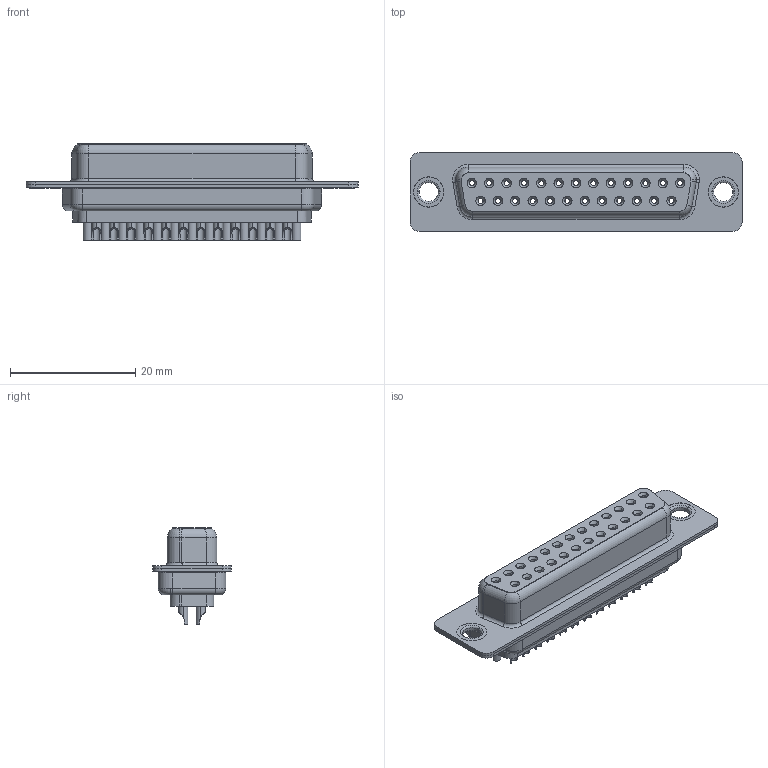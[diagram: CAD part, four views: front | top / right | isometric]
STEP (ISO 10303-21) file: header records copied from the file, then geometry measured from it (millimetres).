
FILE_DESCRIPTION (( 'STEP AP203' ), '1' );
FILE_NAME ('628-025-622-061.STEP', '2020-07-14T15:30:57', ( '' ), ( '' ), 'SwSTEP 2.0', 'SolidWorks 2020', '' );
FILE_SCHEMA (( 'CONFIG_CONTROL_DESIGN' ));
Length unit declared in the file: millimetre
Products named in the file (7): 628 Thru Hole Rivet; 628 Contact Row 2_22L; 628 Housing_25 LP; 628-025-622-061; 628 Contact Row 1_22L; 628 Shell Front_25 Contacts; 628 Shell Rear_25 Contacts
Assembly tree (30 placements, depth 2):
  628-025-622-061
    628 Housing_25 LP
    628 Shell Front_25 Contacts
    628 Shell Rear_25 Contacts
    628 Contact Row 1_22L  x13
    628 Contact Row 2_22L  x12
    628 Thru Hole Rivet  x2
Bounding box: 53 x 12.6 x 15.35 mm (x, y, z)
Volume: 3766.9 mm3; surface area: 9245.1 mm2
Topology: 30 solids, 30 shells, 2478 faces, 6253 edges, 3921 vertices
Faces by surface type: cylinder 746, plane 592, torus 515, bspline 500, cone 125
Entity records: 23613 total; most frequent: CARTESIAN_POINT 5547, DIRECTION 3731, ORIENTED_EDGE 3318, EDGE_CURVE 1659, AXIS2_PLACEMENT_3D 1568, VERTEX_POINT 1045, CIRCLE 865, EDGE_LOOP 858
